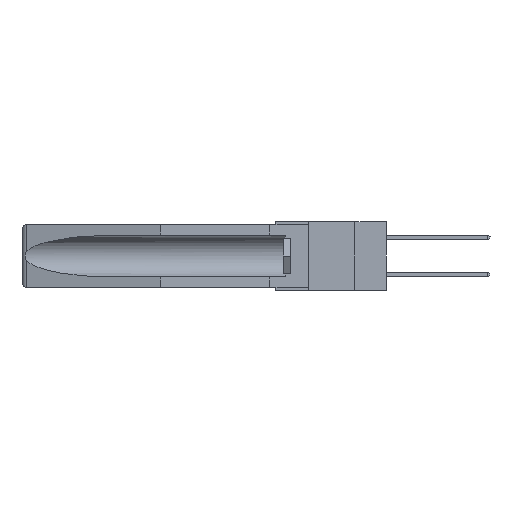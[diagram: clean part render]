
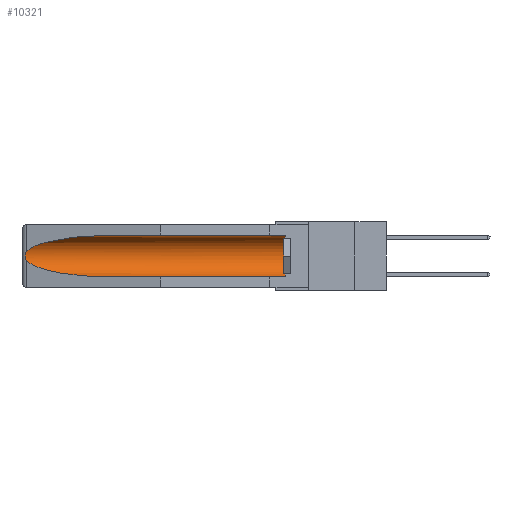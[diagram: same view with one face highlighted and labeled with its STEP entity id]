
A CAD part, left-side view. The second image highlights one B-rep face of the part: STEP entity #10321.
In plain terms, the highlighted cylindrical face has radius 2.857 mm (diameter 5.715 mm), a partial arc.
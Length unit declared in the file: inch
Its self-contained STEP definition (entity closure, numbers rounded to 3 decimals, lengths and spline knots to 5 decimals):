
#18 = CARTESIAN_POINT ( 'NONE',  ( 0.26537, 1.52718, -0.19328 ) ) ;
#820 = DIRECTION ( 'NONE',  ( 0., 1., 0. ) ) ;
#1054 = EDGE_CURVE ( 'NONE', #25206, #17189, #22214, .T. ) ;
#1245 = DIRECTION ( 'NONE',  ( 0., 1., 0. ) ) ;
#1882 = CARTESIAN_POINT ( 'NONE',  ( 0.2675, 1.53308, -0.17534 ) ) ;
#1909 = EDGE_CURVE ( 'NONE', #8391, #15826, #24462, .T. ) ;
#2345 = CARTESIAN_POINT ( 'NONE',  ( 0.155, 1.07973, -0.284 ) ) ;
#3709 = CARTESIAN_POINT ( 'NONE',  ( 0.155, -0.30754, -0.284 ) ) ;
#3874 = CARTESIAN_POINT ( 'NONE',  ( 0.26597, 1.5296, -0.19026 ) ) ;
#4551 = CARTESIAN_POINT ( 'NONE',  ( 0.25451, 1.48313, -0.24835 ) ) ;
#5520 = CARTESIAN_POINT ( 'NONE',  ( 0.155, 0.126, -0.1715 ) ) ;
#5620 = DIRECTION ( 'NONE',  ( 0., -1., 0. ) ) ;
#5792 = CARTESIAN_POINT ( 'NONE',  ( 0.155, -0.30754, -0.059 ) ) ;
#6222 = CARTESIAN_POINT ( 'NONE',  ( 0.155, 1.07973, -0.059 ) ) ;
#7014 = EDGE_CURVE ( 'NONE', #17189, #8391, #29098, .T. ) ;
#7814 = DIRECTION ( 'NONE',  ( 0., 0., 1. ) ) ;
#7912 = CARTESIAN_POINT ( 'NONE',  ( 0.155, -0.30754, -0.1715 ) ) ;
#8329 = LINE ( 'NONE', #3709, #16340 ) ;
#8391 = VERTEX_POINT ( 'NONE', #20918 ) ;
#8475 = CARTESIAN_POINT ( 'NONE',  ( 0.26597, 1.52961, -0.15275 ) ) ;
#8552 = ORIENTED_EDGE ( 'NONE', *, *, #7014, .T. ) ;
#8677 = CARTESIAN_POINT ( 'NONE',  ( 0.2673, 1.53269, -0.17917 ) ) ;
#8882 = CARTESIAN_POINT ( 'NONE',  ( 0.2673, 1.5327, -0.16383 ) ) ;
#8937 = CARTESIAN_POINT ( 'NONE',  ( 0.155, 0.126, -0.284 ) ) ;
#9623 = ORIENTED_EDGE ( 'NONE', *, *, #1054, .T. ) ;
#10321 = ADVANCED_FACE ( 'NONE', ( #16184 ), #18368, .F. ) ;
#10396 = CIRCLE ( 'NONE', #20104, 0.1125 ) ;
#10913 = CARTESIAN_POINT ( 'NONE',  ( 0.21114, 1.30732, -0.059 ) ) ;
#11523 = AXIS2_PLACEMENT_3D ( 'NONE', #7912, #820, #7814 ) ;
#13094 = CARTESIAN_POINT ( 'NONE',  ( 0.26654, 1.53092, -0.15636 ) ) ;
#13331 = EDGE_CURVE ( 'NONE', #18306, #15178, #10396, .T. ) ;
#13377 = CARTESIAN_POINT ( 'NONE',  ( 0.26537, 1.52718, -0.19328 ) ) ;
#13391 = CARTESIAN_POINT ( 'NONE',  ( 0.26537, 1.52718, -0.14972 ) ) ;
#14771 = CARTESIAN_POINT ( 'NONE',  ( 0.155, 1.07973, -0.059 ) ) ;
#15069 = EDGE_CURVE ( 'NONE', #15178, #25206, #22225, .T. ) ;
#15178 = VERTEX_POINT ( 'NONE', #21983 ) ;
#15585 = CARTESIAN_POINT ( 'NONE',  ( 0.25451, 1.48313, -0.09465 ) ) ;
#15826 = VERTEX_POINT ( 'NONE', #26903 ) ;
#16184 = FACE_OUTER_BOUND ( 'NONE', #25874, .T. ) ;
#16272 = CARTESIAN_POINT ( 'NONE',  ( 0.21114, 1.30732, -0.284 ) ) ;
#16340 = VECTOR ( 'NONE', #1245, 39.37008 ) ;
#17189 = VERTEX_POINT ( 'NONE', #13391 ) ;
#17713 = ORIENTED_EDGE ( 'NONE', *, *, #1909, .T. ) ;
#18306 = VERTEX_POINT ( 'NONE', #8937 ) ;
#18368 = CYLINDRICAL_SURFACE ( 'NONE', #11523, 0.1125 ) ;
#20104 = AXIS2_PLACEMENT_3D ( 'NONE', #5520, #5620, #28464 ) ;
#20129 = ORIENTED_EDGE ( 'NONE', *, *, #13331, .T. ) ;
#20918 = CARTESIAN_POINT ( 'NONE',  ( 0.26537, 1.52718, -0.19328 ) ) ;
#21026 = ORIENTED_EDGE ( 'NONE', *, *, #15069, .T. ) ;
#21983 = CARTESIAN_POINT ( 'NONE',  ( 0.155, 0.126, -0.059 ) ) ;
#22214 =( BOUNDED_CURVE ( )  B_SPLINE_CURVE ( 3, ( #6222, #10913, #15585, #22539 ),
 .UNSPECIFIED., .F., .F. ) 
 B_SPLINE_CURVE_WITH_KNOTS ( ( 4, 4 ),
 ( 4.71239, 6.08839 ),
 .UNSPECIFIED. ) 
 CURVE ( )  GEOMETRIC_REPRESENTATION_ITEM ( )  RATIONAL_B_SPLINE_CURVE ( ( 1., 0.848, 0.848, 1. ) ) 
 REPRESENTATION_ITEM ( '' )  );
#22225 = LINE ( 'NONE', #5792, #23681 ) ;
#22334 = ORIENTED_EDGE ( 'NONE', *, *, #28702, .F. ) ;
#22539 = CARTESIAN_POINT ( 'NONE',  ( 0.26537, 1.52718, -0.14972 ) ) ;
#22558 = CARTESIAN_POINT ( 'NONE',  ( 0.2675, 1.53308, -0.16763 ) ) ;
#23681 = VECTOR ( 'NONE', #26200, 39.37008 ) ;
#24462 =( BOUNDED_CURVE ( )  B_SPLINE_CURVE ( 3, ( #18, #4551, #16272, #2345 ),
 .UNSPECIFIED., .F., .F. ) 
 B_SPLINE_CURVE_WITH_KNOTS ( ( 4, 4 ),
 ( 0.1948, 1.5708 ),
 .UNSPECIFIED. ) 
 CURVE ( )  GEOMETRIC_REPRESENTATION_ITEM ( )  RATIONAL_B_SPLINE_CURVE ( ( 1., 0.848, 0.848, 1. ) ) 
 REPRESENTATION_ITEM ( '' )  );
#24731 = CARTESIAN_POINT ( 'NONE',  ( 0.26655, 1.53094, -0.18657 ) ) ;
#25206 = VERTEX_POINT ( 'NONE', #14771 ) ;
#25874 = EDGE_LOOP ( 'NONE', ( #9623, #8552, #17713, #22334, #20129, #21026 ) ) ;
#26200 = DIRECTION ( 'NONE',  ( 0., 1., 0. ) ) ;
#26903 = CARTESIAN_POINT ( 'NONE',  ( 0.155, 1.07973, -0.284 ) ) ;
#28464 = DIRECTION ( 'NONE',  ( 0., 0., 1. ) ) ;
#28702 = EDGE_CURVE ( 'NONE', #18306, #15826, #8329, .T. ) ;
#29098 = B_SPLINE_CURVE_WITH_KNOTS ( 'NONE', 3,
 ( #29479, #8475, #13094, #8882, #22558, #1882, #8677, #24731, #3874, #13377 ),
 .UNSPECIFIED., .F., .F.,
 ( 4, 2, 2, 2, 4 ),
 ( 0., 0.00029, 0.00058, 0.00087, 0.00117 ),
 .UNSPECIFIED. ) ;
#29479 = CARTESIAN_POINT ( 'NONE',  ( 0.26537, 1.52718, -0.14972 ) ) ;
